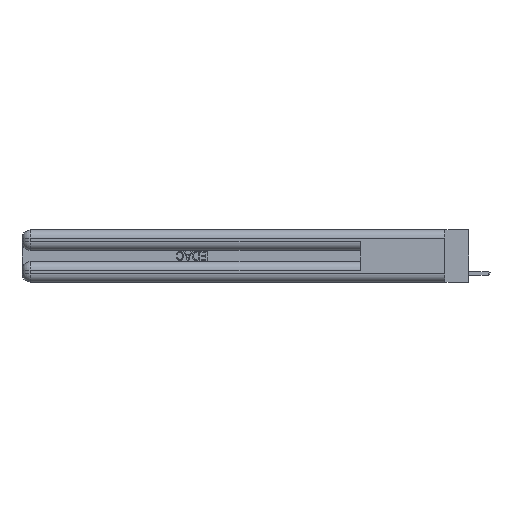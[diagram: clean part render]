
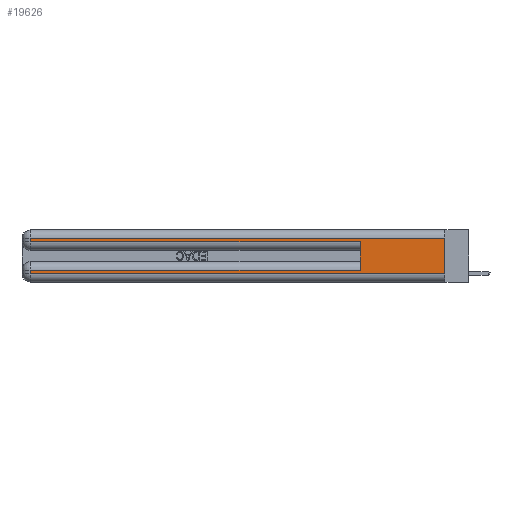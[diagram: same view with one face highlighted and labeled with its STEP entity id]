
A CAD part, left-side view. The second image highlights one B-rep face of the part: STEP entity #19626.
In plain terms, the highlighted planar face has unit normal (-1, 0, 0).
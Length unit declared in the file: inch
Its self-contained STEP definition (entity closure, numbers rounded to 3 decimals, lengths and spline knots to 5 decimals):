
#314 = DIRECTION ( 'NONE',  ( 0., 1., 0. ) ) ;
#492 = DIRECTION ( 'NONE',  ( 0., -1., 0. ) ) ;
#695 = EDGE_CURVE ( 'NONE', #17562, #11543, #12711, .T. ) ;
#858 = CARTESIAN_POINT ( 'NONE',  ( 0., 0.6, 0.145 ) ) ;
#1203 = CARTESIAN_POINT ( 'NONE',  ( 0., 0., 0.37 ) ) ;
#1591 = DIRECTION ( 'NONE',  ( 0., 0., -1. ) ) ;
#2195 = DIRECTION ( 'NONE',  ( 0., 0., -1. ) ) ;
#2258 = CARTESIAN_POINT ( 'NONE',  ( 0., 2.94, 0.37 ) ) ;
#3335 = ORIENTED_EDGE ( 'NONE', *, *, #16735, .T. ) ;
#4095 = EDGE_CURVE ( 'NONE', #17562, #9142, #12206, .T. ) ;
#4469 = CARTESIAN_POINT ( 'NONE',  ( 0., 0.6, 0.085 ) ) ;
#4514 = EDGE_CURVE ( 'NONE', #5239, #8342, #26008, .T. ) ;
#4752 = VECTOR ( 'NONE', #17323, 39.37008 ) ;
#5090 = CARTESIAN_POINT ( 'NONE',  ( 0., 2.94, 0.085 ) ) ;
#5239 = VERTEX_POINT ( 'NONE', #5090 ) ;
#6092 = FACE_OUTER_BOUND ( 'NONE', #24550, .T. ) ;
#6452 = ORIENTED_EDGE ( 'NONE', *, *, #23420, .T. ) ;
#7532 = DIRECTION ( 'NONE',  ( 1., 0., 0. ) ) ;
#7593 = EDGE_CURVE ( 'NONE', #24560, #12723, #15403, .T. ) ;
#7628 = VECTOR ( 'NONE', #1591, 39.37008 ) ;
#7875 = VECTOR ( 'NONE', #2195, 39.37008 ) ;
#8117 = ORIENTED_EDGE ( 'NONE', *, *, #4095, .T. ) ;
#8192 = AXIS2_PLACEMENT_3D ( 'NONE', #1203, #7532, #16308 ) ;
#8342 = VERTEX_POINT ( 'NONE', #9570 ) ;
#8720 = CARTESIAN_POINT ( 'NONE',  ( 0., 2.94, 0.31 ) ) ;
#9142 = VERTEX_POINT ( 'NONE', #8720 ) ;
#9570 = CARTESIAN_POINT ( 'NONE',  ( 0., 2.94, 0.06 ) ) ;
#9928 = ORIENTED_EDGE ( 'NONE', *, *, #7593, .T. ) ;
#10021 = ORIENTED_EDGE ( 'NONE', *, *, #695, .F. ) ;
#10288 = CARTESIAN_POINT ( 'NONE',  ( 0., 0., 0.31 ) ) ;
#11157 = CARTESIAN_POINT ( 'NONE',  ( 0., 0., 0.085 ) ) ;
#11220 = VERTEX_POINT ( 'NONE', #4469 ) ;
#11251 = DIRECTION ( 'NONE',  ( 0., 1., 0. ) ) ;
#11287 = CARTESIAN_POINT ( 'NONE',  ( 0., 0., 0.37 ) ) ;
#11292 = EDGE_CURVE ( 'NONE', #9142, #24560, #24084, .T. ) ;
#11543 = VERTEX_POINT ( 'NONE', #12243 ) ;
#12206 = LINE ( 'NONE', #13266, #18910 ) ;
#12243 = CARTESIAN_POINT ( 'NONE',  ( 0., 0., 0.06 ) ) ;
#12711 = LINE ( 'NONE', #11287, #7628 ) ;
#12723 = VERTEX_POINT ( 'NONE', #25549 ) ;
#13266 = CARTESIAN_POINT ( 'NONE',  ( 0., 0., 0.31 ) ) ;
#14002 = VECTOR ( 'NONE', #11251, 39.37008 ) ;
#14164 = PLANE ( 'NONE',  #8192 ) ;
#15137 = CARTESIAN_POINT ( 'NONE',  ( 0., 2.94, 0.37 ) ) ;
#15403 = LINE ( 'NONE', #24226, #17400 ) ;
#15616 = DIRECTION ( 'NONE',  ( 0., 0., 1. ) ) ;
#15921 = CARTESIAN_POINT ( 'NONE',  ( 0., 2.94, 0.285 ) ) ;
#16308 = DIRECTION ( 'NONE',  ( 0., 0., -1. ) ) ;
#16735 = EDGE_CURVE ( 'NONE', #8342, #11543, #18380, .T. ) ;
#17229 = VECTOR ( 'NONE', #15616, 39.37008 ) ;
#17323 = DIRECTION ( 'NONE',  ( 0., 0., -1. ) ) ;
#17400 = VECTOR ( 'NONE', #492, 39.37008 ) ;
#17562 = VERTEX_POINT ( 'NONE', #10288 ) ;
#18380 = LINE ( 'NONE', #20229, #22826 ) ;
#18910 = VECTOR ( 'NONE', #314, 39.37008 ) ;
#18992 = EDGE_CURVE ( 'NONE', #11220, #12723, #25718, .T. ) ;
#19626 = ADVANCED_FACE ( 'NONE', ( #6092 ), #14164, .F. ) ;
#20229 = CARTESIAN_POINT ( 'NONE',  ( 0., 0., 0.06 ) ) ;
#22826 = VECTOR ( 'NONE', #26756, 39.37008 ) ;
#22884 = ORIENTED_EDGE ( 'NONE', *, *, #18992, .F. ) ;
#22947 = ORIENTED_EDGE ( 'NONE', *, *, #11292, .T. ) ;
#23420 = EDGE_CURVE ( 'NONE', #11220, #5239, #27169, .T. ) ;
#24084 = LINE ( 'NONE', #15137, #7875 ) ;
#24226 = CARTESIAN_POINT ( 'NONE',  ( 0., 0., 0.285 ) ) ;
#24550 = EDGE_LOOP ( 'NONE', ( #10021, #8117, #22947, #9928, #22884, #6452, #25975, #3335 ) ) ;
#24560 = VERTEX_POINT ( 'NONE', #15921 ) ;
#25549 = CARTESIAN_POINT ( 'NONE',  ( 0., 0.6, 0.285 ) ) ;
#25718 = LINE ( 'NONE', #858, #17229 ) ;
#25975 = ORIENTED_EDGE ( 'NONE', *, *, #4514, .T. ) ;
#26008 = LINE ( 'NONE', #2258, #4752 ) ;
#26756 = DIRECTION ( 'NONE',  ( 0., -1., 0. ) ) ;
#27169 = LINE ( 'NONE', #11157, #14002 ) ;
